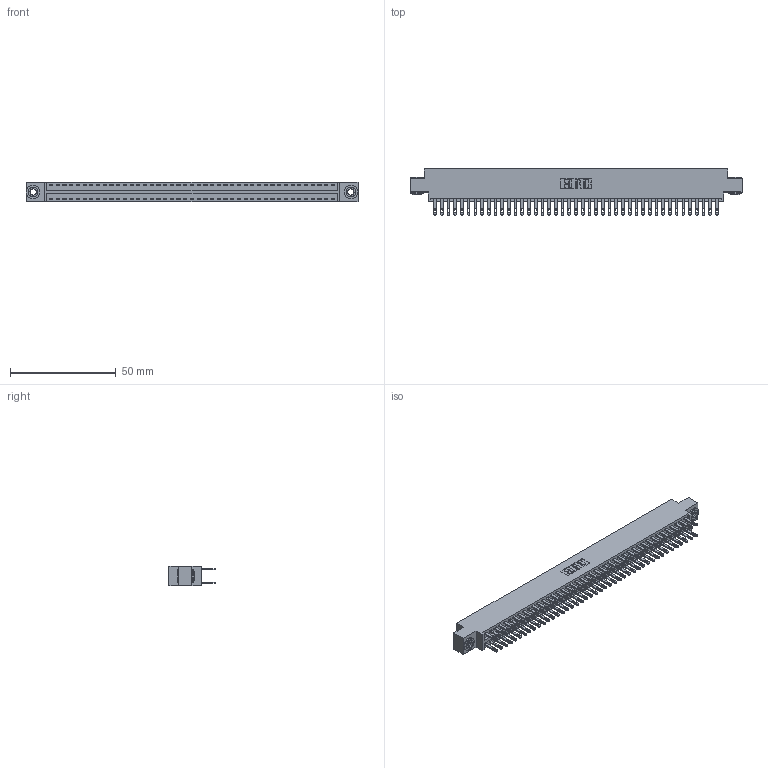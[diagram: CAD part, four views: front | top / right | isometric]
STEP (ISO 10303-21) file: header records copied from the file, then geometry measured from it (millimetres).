
FILE_DESCRIPTION (( 'STEP AP203' ), '1' );
FILE_NAME ('896-086-500-803.STEP', '2021-07-28T02:35:49', ( '' ), ( '' ), 'SwSTEP 2.0', 'SolidWorks 2020', '' );
FILE_SCHEMA (( 'CONFIG_CONTROL_DESIGN' ));
Length unit declared in the file: inch
Products named in the file (4): 896-086-500-803; 345-292-001_345-293-100; 345-250-002_345-250-002-102; 846 Part_0.170 Offset - 0.156 Dia-TH
Assembly tree (89 placements, depth 2):
  896-086-500-803
    846 Part_0.170 Offset - 0.156 Dia-TH
    345-292-001_345-293-100  x86
    345-250-002_345-250-002-102  x2
Bounding box: 157.1 x 21.84 x 9.4 mm (x, y, z)
Volume: 15454.5 mm3; surface area: 22552.8 mm2
Topology: 89 solids, 89 shells, 4292 faces, 13059 edges, 8702 vertices
Faces by surface type: plane 2584, cylinder 1700, cone 8
Entity records: 28640 total; most frequent: CARTESIAN_POINT 4695, ORIENTED_EDGE 4622, DIRECTION 4221, EDGE_CURVE 2311, VECTOR 1979, LINE 1979, VERTEX_POINT 1538, AXIS2_PLACEMENT_3D 1121
